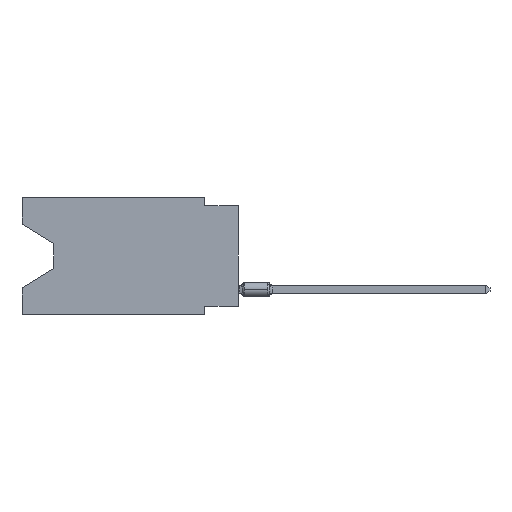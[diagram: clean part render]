
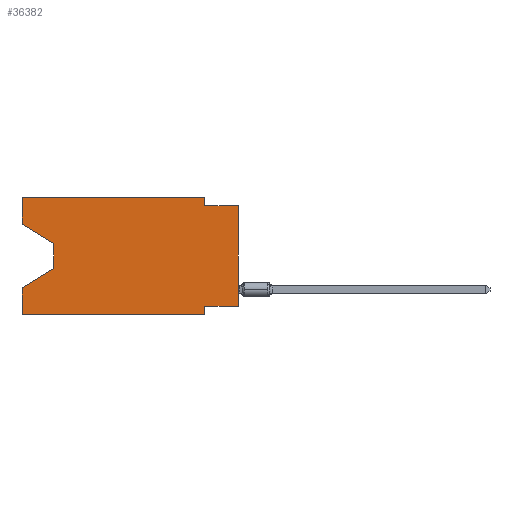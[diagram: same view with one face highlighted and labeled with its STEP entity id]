
A CAD part, left-side view. The second image highlights one B-rep face of the part: STEP entity #36382.
In plain terms, the highlighted planar face has unit normal (-1, 0, 0).
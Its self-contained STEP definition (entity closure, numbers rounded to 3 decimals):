
#726 = CARTESIAN_POINT ( 'NONE',  ( 0., 13.97, -3.505 ) ) ;
#1088 = DIRECTION ( 'NONE',  ( 0., 0., 1. ) ) ;
#1263 = ORIENTED_EDGE ( 'NONE', *, *, #21239, .T. ) ;
#1296 = LINE ( 'NONE', #36881, #34071 ) ;
#1574 = DIRECTION ( 'NONE',  ( 0., 0., -1. ) ) ;
#2299 = ORIENTED_EDGE ( 'NONE', *, *, #10532, .F. ) ;
#2313 = CARTESIAN_POINT ( 'NONE',  ( 0., 16.383, 0. ) ) ;
#2422 = CARTESIAN_POINT ( 'NONE',  ( 0., 16.383, 0. ) ) ;
#2626 = VECTOR ( 'NONE', #12212, 1000. ) ;
#2731 = ORIENTED_EDGE ( 'NONE', *, *, #21536, .T. ) ;
#3255 = EDGE_CURVE ( 'NONE', #14972, #39739, #32557, .T. ) ;
#3378 = DIRECTION ( 'NONE',  ( 0., 0., 1. ) ) ;
#4649 = ORIENTED_EDGE ( 'NONE', *, *, #6810, .F. ) ;
#4766 = CARTESIAN_POINT ( 'NONE',  ( 0., 16.383, -2.038 ) ) ;
#5259 = VERTEX_POINT ( 'NONE', #26290 ) ;
#5399 = PLANE ( 'NONE',  #14103 ) ;
#6293 = EDGE_CURVE ( 'NONE', #31006, #40445, #12114, .T. ) ;
#6300 = DIRECTION ( 'NONE',  ( 0., 0., -1. ) ) ;
#6450 = CARTESIAN_POINT ( 'NONE',  ( 0., 0., -0.635 ) ) ;
#6653 = EDGE_CURVE ( 'NONE', #14972, #30284, #33961, .T. ) ;
#6810 = EDGE_CURVE ( 'NONE', #12186, #31823, #10499, .T. ) ;
#8432 = ORIENTED_EDGE ( 'NONE', *, *, #39292, .F. ) ;
#8600 = VECTOR ( 'NONE', #39453, 1000. ) ;
#8887 = DIRECTION ( 'NONE',  ( 0., 0., -1. ) ) ;
#9198 = DIRECTION ( 'NONE',  ( 0., 0., -1. ) ) ;
#9489 = LINE ( 'NONE', #26093, #23504 ) ;
#9534 = ORIENTED_EDGE ( 'NONE', *, *, #26870, .F. ) ;
#10485 = EDGE_CURVE ( 'NONE', #32810, #26988, #40980, .T. ) ;
#10499 = LINE ( 'NONE', #20068, #8600 ) ;
#10532 = EDGE_CURVE ( 'NONE', #5259, #13464, #35200, .T. ) ;
#10635 = LINE ( 'NONE', #2313, #13101 ) ;
#12074 = ORIENTED_EDGE ( 'NONE', *, *, #22024, .F. ) ;
#12114 = LINE ( 'NONE', #19123, #30329 ) ;
#12186 = VERTEX_POINT ( 'NONE', #31061 ) ;
#12212 = DIRECTION ( 'NONE',  ( 0., 0.855, -0.519 ) ) ;
#13101 = VECTOR ( 'NONE', #21041, 1000. ) ;
#13464 = VERTEX_POINT ( 'NONE', #6450 ) ;
#14103 = AXIS2_PLACEMENT_3D ( 'NONE', #19211, #15398, #9198 ) ;
#14972 = VERTEX_POINT ( 'NONE', #22097 ) ;
#14994 = DIRECTION ( 'NONE',  ( 0., -1., 0. ) ) ;
#15220 = LINE ( 'NONE', #2422, #19022 ) ;
#15292 = LINE ( 'NONE', #41266, #15722 ) ;
#15398 = DIRECTION ( 'NONE',  ( 1., 0., 0. ) ) ;
#15719 = CARTESIAN_POINT ( 'NONE',  ( 0., 16.383, 0. ) ) ;
#15722 = VECTOR ( 'NONE', #8887, 1000. ) ;
#16378 = CARTESIAN_POINT ( 'NONE',  ( 0., 16.383, 0. ) ) ;
#16661 = ORIENTED_EDGE ( 'NONE', *, *, #34215, .F. ) ;
#16877 = CARTESIAN_POINT ( 'NONE',  ( 0., 2.54, -8.89 ) ) ;
#19022 = VECTOR ( 'NONE', #34391, 1000. ) ;
#19123 = CARTESIAN_POINT ( 'NONE',  ( 0., 16.383, -8.89 ) ) ;
#19211 = CARTESIAN_POINT ( 'NONE',  ( 0., 16.383, 0. ) ) ;
#20068 = CARTESIAN_POINT ( 'NONE',  ( 0., 0., -8.255 ) ) ;
#21041 = DIRECTION ( 'NONE',  ( 0., -1., 0. ) ) ;
#21239 = EDGE_CURVE ( 'NONE', #30284, #32810, #26709, .T. ) ;
#21536 = EDGE_CURVE ( 'NONE', #12186, #13464, #1296, .T. ) ;
#22024 = EDGE_CURVE ( 'NONE', #39739, #24009, #10635, .T. ) ;
#22097 = CARTESIAN_POINT ( 'NONE',  ( 0., 16.383, -2.038 ) ) ;
#23255 = VECTOR ( 'NONE', #3378, 1000. ) ;
#23504 = VECTOR ( 'NONE', #6300, 1000. ) ;
#23559 = ORIENTED_EDGE ( 'NONE', *, *, #6653, .T. ) ;
#23848 = EDGE_LOOP ( 'NONE', ( #23559, #1263, #42076, #8432, #31558, #16661, #4649, #2731, #2299, #9534, #12074, #35685 ) ) ;
#24009 = VERTEX_POINT ( 'NONE', #36808 ) ;
#24484 = CARTESIAN_POINT ( 'NONE',  ( 0., 2.54, -8.255 ) ) ;
#25089 = DIRECTION ( 'NONE',  ( 0., -1., 0. ) ) ;
#25190 = CARTESIAN_POINT ( 'NONE',  ( 0., 0., -0.635 ) ) ;
#26093 = CARTESIAN_POINT ( 'NONE',  ( 0., 2.54, 0. ) ) ;
#26290 = CARTESIAN_POINT ( 'NONE',  ( 0., 2.54, -0.635 ) ) ;
#26709 = LINE ( 'NONE', #726, #39510 ) ;
#26870 = EDGE_CURVE ( 'NONE', #24009, #5259, #9489, .T. ) ;
#26988 = VERTEX_POINT ( 'NONE', #30989 ) ;
#28426 = CARTESIAN_POINT ( 'NONE',  ( 0., 16.383, -8.89 ) ) ;
#30284 = VERTEX_POINT ( 'NONE', #38726 ) ;
#30329 = VECTOR ( 'NONE', #25089, 1000. ) ;
#30776 = DIRECTION ( 'NONE',  ( 0., -0.855, -0.519 ) ) ;
#30989 = CARTESIAN_POINT ( 'NONE',  ( 0., 16.383, -6.852 ) ) ;
#31006 = VERTEX_POINT ( 'NONE', #28426 ) ;
#31061 = CARTESIAN_POINT ( 'NONE',  ( 0., 0., -8.255 ) ) ;
#31558 = ORIENTED_EDGE ( 'NONE', *, *, #6293, .T. ) ;
#31823 = VERTEX_POINT ( 'NONE', #24484 ) ;
#32557 = LINE ( 'NONE', #16378, #23255 ) ;
#32810 = VERTEX_POINT ( 'NONE', #39992 ) ;
#33961 = LINE ( 'NONE', #4766, #40554 ) ;
#34071 = VECTOR ( 'NONE', #1088, 1000. ) ;
#34215 = EDGE_CURVE ( 'NONE', #31823, #40445, #15292, .T. ) ;
#34391 = DIRECTION ( 'NONE',  ( 0., 0., 1. ) ) ;
#35200 = LINE ( 'NONE', #25190, #36634 ) ;
#35685 = ORIENTED_EDGE ( 'NONE', *, *, #3255, .F. ) ;
#36382 = ADVANCED_FACE ( 'NONE', ( #37779 ), #5399, .F. ) ;
#36634 = VECTOR ( 'NONE', #14994, 1000. ) ;
#36808 = CARTESIAN_POINT ( 'NONE',  ( 0., 2.54, 0. ) ) ;
#36881 = CARTESIAN_POINT ( 'NONE',  ( 0., 0., 0. ) ) ;
#37779 = FACE_OUTER_BOUND ( 'NONE', #23848, .T. ) ;
#38400 = CARTESIAN_POINT ( 'NONE',  ( 0., 13.97, -5.385 ) ) ;
#38726 = CARTESIAN_POINT ( 'NONE',  ( 0., 13.97, -3.505 ) ) ;
#39292 = EDGE_CURVE ( 'NONE', #31006, #26988, #15220, .T. ) ;
#39453 = DIRECTION ( 'NONE',  ( 0., 1., 0. ) ) ;
#39510 = VECTOR ( 'NONE', #1574, 1000. ) ;
#39739 = VERTEX_POINT ( 'NONE', #15719 ) ;
#39992 = CARTESIAN_POINT ( 'NONE',  ( 0., 13.97, -5.385 ) ) ;
#40445 = VERTEX_POINT ( 'NONE', #16877 ) ;
#40554 = VECTOR ( 'NONE', #30776, 1000. ) ;
#40980 = LINE ( 'NONE', #38400, #2626 ) ;
#41266 = CARTESIAN_POINT ( 'NONE',  ( 0., 2.54, -8.89 ) ) ;
#42076 = ORIENTED_EDGE ( 'NONE', *, *, #10485, .T. ) ;
